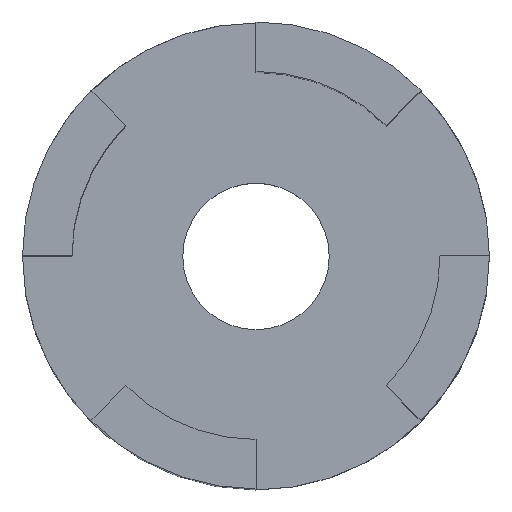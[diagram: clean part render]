
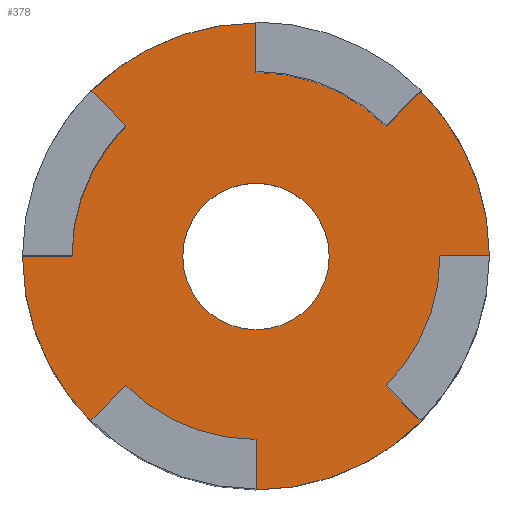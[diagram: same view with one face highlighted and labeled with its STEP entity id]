
A CAD part, top view. The second image highlights one B-rep face of the part: STEP entity #378.
In plain terms, the highlighted planar face has unit normal (0, 0, 1).
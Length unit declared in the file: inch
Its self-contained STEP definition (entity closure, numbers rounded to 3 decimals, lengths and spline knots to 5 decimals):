
#15=FACE_BOUND('',#65,.T.);
#26=PLANE('',#430);
#44=FACE_OUTER_BOUND('',#64,.T.);
#64=EDGE_LOOP('',(#304,#305,#306,#307,#308,#309,#310,#311,#312,#313,#314,
#315,#316,#317,#318,#319));
#65=EDGE_LOOP('',(#320));
#74=LINE('',#573,#108);
#79=LINE('',#587,#113);
#82=LINE('',#596,#116);
#87=LINE('',#610,#121);
#90=LINE('',#619,#124);
#95=LINE('',#633,#129);
#98=LINE('',#643,#132);
#99=LINE('',#647,#133);
#108=VECTOR('',#458,0.3937);
#113=VECTOR('',#471,0.3937);
#116=VECTOR('',#480,0.3937);
#121=VECTOR('',#493,0.3937);
#124=VECTOR('',#502,0.3937);
#129=VECTOR('',#515,0.3937);
#132=VECTOR('',#526,0.3937);
#133=VECTOR('',#529,0.3937);
#143=CIRCLE('',#408,0.1255);
#144=CIRCLE('',#411,0.31535);
#147=CIRCLE('',#418,0.31535);
#150=CIRCLE('',#425,0.31535);
#153=CIRCLE('',#431,0.4);
#154=CIRCLE('',#432,0.31535);
#155=CIRCLE('',#433,0.4);
#156=CIRCLE('',#434,0.4);
#157=CIRCLE('',#435,0.4);
#163=VERTEX_POINT('',#567);
#164=VERTEX_POINT('',#571);
#165=VERTEX_POINT('',#572);
#168=VERTEX_POINT('',#580);
#170=VERTEX_POINT('',#586);
#172=VERTEX_POINT('',#594);
#173=VERTEX_POINT('',#595);
#176=VERTEX_POINT('',#603);
#178=VERTEX_POINT('',#609);
#180=VERTEX_POINT('',#617);
#181=VERTEX_POINT('',#618);
#184=VERTEX_POINT('',#626);
#186=VERTEX_POINT('',#632);
#188=VERTEX_POINT('',#640);
#189=VERTEX_POINT('',#642);
#190=VERTEX_POINT('',#644);
#191=VERTEX_POINT('',#646);
#200=EDGE_CURVE('',#163,#163,#143,.T.);
#201=EDGE_CURVE('',#164,#165,#74,.T.);
#205=EDGE_CURVE('',#165,#168,#144,.T.);
#208=EDGE_CURVE('',#168,#170,#79,.T.);
#212=EDGE_CURVE('',#172,#173,#82,.T.);
#216=EDGE_CURVE('',#173,#176,#147,.T.);
#219=EDGE_CURVE('',#176,#178,#87,.T.);
#223=EDGE_CURVE('',#180,#181,#90,.T.);
#227=EDGE_CURVE('',#181,#184,#150,.T.);
#230=EDGE_CURVE('',#184,#186,#95,.T.);
#234=EDGE_CURVE('',#170,#188,#153,.T.);
#235=EDGE_CURVE('',#188,#189,#98,.T.);
#236=EDGE_CURVE('',#189,#190,#154,.T.);
#237=EDGE_CURVE('',#190,#191,#99,.T.);
#238=EDGE_CURVE('',#191,#180,#155,.T.);
#239=EDGE_CURVE('',#186,#172,#156,.T.);
#240=EDGE_CURVE('',#178,#164,#157,.T.);
#304=ORIENTED_EDGE('',*,*,#201,.T.);
#305=ORIENTED_EDGE('',*,*,#205,.T.);
#306=ORIENTED_EDGE('',*,*,#208,.T.);
#307=ORIENTED_EDGE('',*,*,#234,.T.);
#308=ORIENTED_EDGE('',*,*,#235,.T.);
#309=ORIENTED_EDGE('',*,*,#236,.T.);
#310=ORIENTED_EDGE('',*,*,#237,.T.);
#311=ORIENTED_EDGE('',*,*,#238,.T.);
#312=ORIENTED_EDGE('',*,*,#223,.T.);
#313=ORIENTED_EDGE('',*,*,#227,.T.);
#314=ORIENTED_EDGE('',*,*,#230,.T.);
#315=ORIENTED_EDGE('',*,*,#239,.T.);
#316=ORIENTED_EDGE('',*,*,#212,.T.);
#317=ORIENTED_EDGE('',*,*,#216,.T.);
#318=ORIENTED_EDGE('',*,*,#219,.T.);
#319=ORIENTED_EDGE('',*,*,#240,.T.);
#320=ORIENTED_EDGE('',*,*,#200,.T.);
#378=ADVANCED_FACE('',(#44,#15),#26,.T.);
#408=AXIS2_PLACEMENT_3D('',#569,#454,#455);
#411=AXIS2_PLACEMENT_3D('',#581,#464,#465);
#418=AXIS2_PLACEMENT_3D('',#604,#486,#487);
#425=AXIS2_PLACEMENT_3D('',#627,#508,#509);
#430=AXIS2_PLACEMENT_3D('',#639,#522,#523);
#431=AXIS2_PLACEMENT_3D('',#641,#524,#525);
#432=AXIS2_PLACEMENT_3D('',#645,#527,#528);
#433=AXIS2_PLACEMENT_3D('',#648,#530,#531);
#434=AXIS2_PLACEMENT_3D('',#649,#532,#533);
#435=AXIS2_PLACEMENT_3D('',#650,#534,#535);
#454=DIRECTION('center_axis',(0.,0.,-1.));
#455=DIRECTION('ref_axis',(-1.,0.,0.));
#458=DIRECTION('',(0.707,0.707,0.));
#464=DIRECTION('center_axis',(0.,0.,1.));
#465=DIRECTION('ref_axis',(0.707,0.707,0.));
#471=DIRECTION('',(0.,-1.,0.));
#480=DIRECTION('',(0.707,-0.707,0.));
#486=DIRECTION('center_axis',(0.,0.,1.));
#487=DIRECTION('ref_axis',(0.707,-0.707,0.));
#493=DIRECTION('',(-1.,0.,0.));
#502=DIRECTION('',(-0.707,-0.707,0.));
#508=DIRECTION('center_axis',(0.,0.,1.));
#509=DIRECTION('ref_axis',(-0.707,-0.707,0.));
#515=DIRECTION('',(0.,1.,0.));
#522=DIRECTION('center_axis',(0.,0.,1.));
#523=DIRECTION('ref_axis',(1.,0.,0.));
#524=DIRECTION('center_axis',(0.,0.,1.));
#525=DIRECTION('ref_axis',(1.,0.,0.));
#526=DIRECTION('',(-0.707,0.707,0.));
#527=DIRECTION('center_axis',(0.,0.,1.));
#528=DIRECTION('ref_axis',(-0.707,0.707,0.));
#529=DIRECTION('',(1.,0.,0.));
#530=DIRECTION('center_axis',(0.,0.,1.));
#531=DIRECTION('ref_axis',(1.,0.,0.));
#532=DIRECTION('center_axis',(0.,0.,1.));
#533=DIRECTION('ref_axis',(1.,0.,0.));
#534=DIRECTION('center_axis',(0.,0.,1.));
#535=DIRECTION('ref_axis',(1.,0.,0.));
#567=CARTESIAN_POINT('',(0.1255,0.,0.1));
#569=CARTESIAN_POINT('Origin',(0.,0.,0.1));
#571=CARTESIAN_POINT('',(-0.28284,-0.28284,0.1));
#572=CARTESIAN_POINT('',(-0.22299,-0.22299,0.1));
#573=CARTESIAN_POINT('',(-0.11149,-0.11149,0.1));
#580=CARTESIAN_POINT('',(0.,-0.31535,0.1));
#581=CARTESIAN_POINT('Origin',(0.,0.,
0.1));
#586=CARTESIAN_POINT('',(0.,-0.4,0.1));
#587=CARTESIAN_POINT('',(0.,-0.2,0.1));
#594=CARTESIAN_POINT('',(-0.28284,0.28284,0.1));
#595=CARTESIAN_POINT('',(-0.22299,0.22299,0.1));
#596=CARTESIAN_POINT('',(-0.11149,0.11149,0.1));
#603=CARTESIAN_POINT('',(-0.31535,0.,0.1));
#604=CARTESIAN_POINT('Origin',(0.,0.,
0.1));
#609=CARTESIAN_POINT('',(-0.4,0.,0.1));
#610=CARTESIAN_POINT('',(-0.2,0.,0.1));
#617=CARTESIAN_POINT('',(0.28284,0.28284,0.1));
#618=CARTESIAN_POINT('',(0.22299,0.22299,0.1));
#619=CARTESIAN_POINT('',(0.11149,0.11149,0.1));
#626=CARTESIAN_POINT('',(0.,0.31535,0.1));
#627=CARTESIAN_POINT('Origin',(0.,0.,
0.1));
#632=CARTESIAN_POINT('',(0.,0.4,0.1));
#633=CARTESIAN_POINT('',(0.,0.2,0.1));
#639=CARTESIAN_POINT('Origin',(0.,0.,
0.1));
#640=CARTESIAN_POINT('',(0.28284,-0.28284,0.1));
#641=CARTESIAN_POINT('Origin',(0.,0.,0.1));
#642=CARTESIAN_POINT('',(0.22299,-0.22299,0.1));
#643=CARTESIAN_POINT('',(0.11149,-0.11149,0.1));
#644=CARTESIAN_POINT('',(0.31535,0.,0.1));
#645=CARTESIAN_POINT('Origin',(0.,0.,
0.1));
#646=CARTESIAN_POINT('',(0.4,0.,0.1));
#647=CARTESIAN_POINT('',(0.2,0.,0.1));
#648=CARTESIAN_POINT('Origin',(0.,0.,0.1));
#649=CARTESIAN_POINT('Origin',(0.,0.,0.1));
#650=CARTESIAN_POINT('Origin',(0.,0.,0.1));
